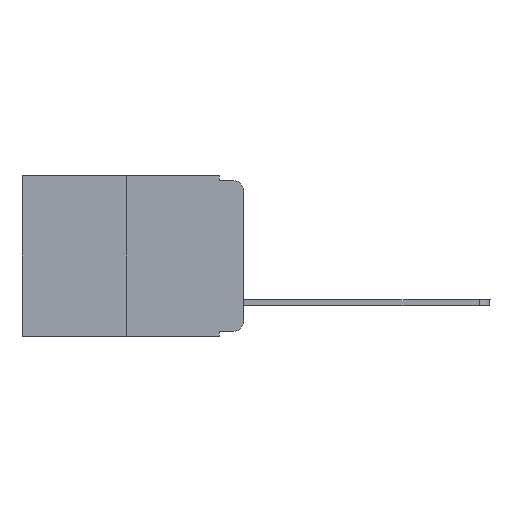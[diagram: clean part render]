
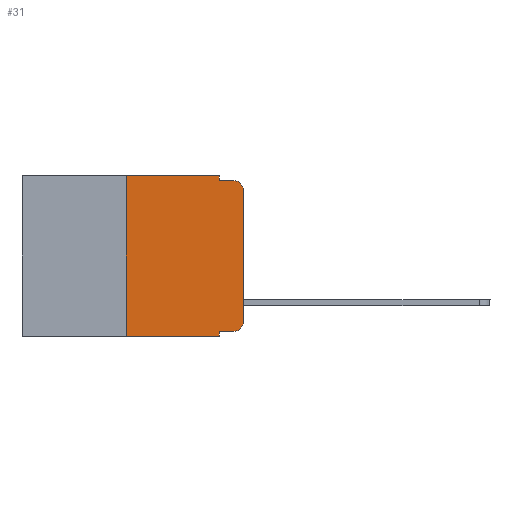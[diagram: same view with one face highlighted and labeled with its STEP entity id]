
A CAD part, left-side view. The second image highlights one B-rep face of the part: STEP entity #31.
In plain terms, the highlighted planar face has unit normal (-1, 0, 0).
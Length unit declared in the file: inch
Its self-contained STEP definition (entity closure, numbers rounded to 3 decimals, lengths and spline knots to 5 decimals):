
#31 = ADVANCED_FACE ( 'NONE', ( #7737 ), #12388, .F. ) ;
#582 = CARTESIAN_POINT ( 'NONE',  ( 0., 0.051, -0.333 ) ) ;
#737 = VECTOR ( 'NONE', #14492, 39.37008 ) ;
#1043 = AXIS2_PLACEMENT_3D ( 'NONE', #17936, #7606, #17555 ) ;
#1588 = VERTEX_POINT ( 'NONE', #3294 ) ;
#1659 = EDGE_CURVE ( 'NONE', #9934, #6963, #11977, .T. ) ;
#2437 = LINE ( 'NONE', #8331, #12179 ) ;
#2709 = VERTEX_POINT ( 'NONE', #6321 ) ;
#2889 = CARTESIAN_POINT ( 'NONE',  ( 0., 0.473, -0.343 ) ) ;
#2942 = EDGE_CURVE ( 'NONE', #1588, #2977, #2437, .T. ) ;
#2977 = VERTEX_POINT ( 'NONE', #8709 ) ;
#3294 = CARTESIAN_POINT ( 'NONE',  ( 0., 0.051, -0.01 ) ) ;
#3409 = EDGE_CURVE ( 'NONE', #14223, #2709, #3972, .T. ) ;
#3478 = CARTESIAN_POINT ( 'NONE',  ( 0., 0., -0.03 ) ) ;
#3717 = CARTESIAN_POINT ( 'NONE',  ( 0., 0.25, 0. ) ) ;
#3972 = LINE ( 'NONE', #8587, #737 ) ;
#4462 = VECTOR ( 'NONE', #11658, 39.37008 ) ;
#4590 = EDGE_LOOP ( 'NONE', ( #5591, #15551, #16948, #12544, #4795, #11921, #11874, #5206, #12717, #8616 ) ) ;
#4795 = ORIENTED_EDGE ( 'NONE', *, *, #3409, .F. ) ;
#4999 = VERTEX_POINT ( 'NONE', #13820 ) ;
#5048 = CARTESIAN_POINT ( 'NONE',  ( 0., 0.473, 0. ) ) ;
#5103 = AXIS2_PLACEMENT_3D ( 'NONE', #16320, #8453, #9553 ) ;
#5129 = VERTEX_POINT ( 'NONE', #3478 ) ;
#5206 = ORIENTED_EDGE ( 'NONE', *, *, #6275, .F. ) ;
#5591 = ORIENTED_EDGE ( 'NONE', *, *, #17825, .T. ) ;
#5823 = EDGE_CURVE ( 'NONE', #11253, #9641, #11933, .T. ) ;
#5833 = CARTESIAN_POINT ( 'NONE',  ( 0., 0.02, -0.333 ) ) ;
#5845 = LINE ( 'NONE', #10463, #8796 ) ;
#6021 = CIRCLE ( 'NONE', #5103, 0.02 ) ;
#6275 = EDGE_CURVE ( 'NONE', #11253, #6963, #5845, .T. ) ;
#6321 = CARTESIAN_POINT ( 'NONE',  ( 0., 0.051, 0. ) ) ;
#6918 = CIRCLE ( 'NONE', #1043, 0.02 ) ;
#6963 = VERTEX_POINT ( 'NONE', #8038 ) ;
#7606 = DIRECTION ( 'NONE',  ( -1., 0., 0. ) ) ;
#7737 = FACE_OUTER_BOUND ( 'NONE', #4590, .T. ) ;
#7942 = DIRECTION ( 'NONE',  ( 1., 0., 0. ) ) ;
#8038 = CARTESIAN_POINT ( 'NONE',  ( 0., 0.051, -0.343 ) ) ;
#8331 = CARTESIAN_POINT ( 'NONE',  ( 0., 0.051, -0.01 ) ) ;
#8453 = DIRECTION ( 'NONE',  ( -1., 0., 0. ) ) ;
#8587 = CARTESIAN_POINT ( 'NONE',  ( 0., 0.473, 0. ) ) ;
#8616 = ORIENTED_EDGE ( 'NONE', *, *, #17842, .T. ) ;
#8709 = CARTESIAN_POINT ( 'NONE',  ( 0., 0.02, -0.01 ) ) ;
#8710 = AXIS2_PLACEMENT_3D ( 'NONE', #5048, #7942, #13839 ) ;
#8762 = CARTESIAN_POINT ( 'NONE',  ( 0., 0., 0. ) ) ;
#8796 = VECTOR ( 'NONE', #10268, 39.37008 ) ;
#9553 = DIRECTION ( 'NONE',  ( 0., 0., -1. ) ) ;
#9641 = VERTEX_POINT ( 'NONE', #5833 ) ;
#9780 = LINE ( 'NONE', #11407, #12116 ) ;
#9934 = VERTEX_POINT ( 'NONE', #17192 ) ;
#10268 = DIRECTION ( 'NONE',  ( 0., 0., -1. ) ) ;
#10463 = CARTESIAN_POINT ( 'NONE',  ( 0., 0.051, 0. ) ) ;
#10466 = DIRECTION ( 'NONE',  ( 0., -1., 0. ) ) ;
#10836 = CARTESIAN_POINT ( 'NONE',  ( 0., 0.051, -0.333 ) ) ;
#11253 = VERTEX_POINT ( 'NONE', #582 ) ;
#11407 = CARTESIAN_POINT ( 'NONE',  ( 0., 0.051, 0. ) ) ;
#11658 = DIRECTION ( 'NONE',  ( 0., 0., 1. ) ) ;
#11874 = ORIENTED_EDGE ( 'NONE', *, *, #1659, .T. ) ;
#11880 = CARTESIAN_POINT ( 'NONE',  ( 0., 0.25, 0. ) ) ;
#11921 = ORIENTED_EDGE ( 'NONE', *, *, #17432, .F. ) ;
#11933 = LINE ( 'NONE', #10836, #13160 ) ;
#11960 = LINE ( 'NONE', #8762, #4462 ) ;
#11977 = LINE ( 'NONE', #2889, #13785 ) ;
#12116 = VECTOR ( 'NONE', #14318, 39.37008 ) ;
#12179 = VECTOR ( 'NONE', #14235, 39.37008 ) ;
#12388 = PLANE ( 'NONE',  #8710 ) ;
#12544 = ORIENTED_EDGE ( 'NONE', *, *, #13841, .F. ) ;
#12717 = ORIENTED_EDGE ( 'NONE', *, *, #5823, .T. ) ;
#13160 = VECTOR ( 'NONE', #10466, 39.37008 ) ;
#13785 = VECTOR ( 'NONE', #14786, 39.37008 ) ;
#13820 = CARTESIAN_POINT ( 'NONE',  ( 0., 0., -0.313 ) ) ;
#13839 = DIRECTION ( 'NONE',  ( 0., 0., -1. ) ) ;
#13841 = EDGE_CURVE ( 'NONE', #2709, #1588, #9780, .T. ) ;
#14223 = VERTEX_POINT ( 'NONE', #3717 ) ;
#14235 = DIRECTION ( 'NONE',  ( 0., -1., 0. ) ) ;
#14318 = DIRECTION ( 'NONE',  ( 0., 0., -1. ) ) ;
#14492 = DIRECTION ( 'NONE',  ( 0., -1., 0. ) ) ;
#14786 = DIRECTION ( 'NONE',  ( 0., -1., 0. ) ) ;
#15551 = ORIENTED_EDGE ( 'NONE', *, *, #18318, .T. ) ;
#16320 = CARTESIAN_POINT ( 'NONE',  ( 0., 0.02, -0.03 ) ) ;
#16412 = DIRECTION ( 'NONE',  ( 0., 0., 1. ) ) ;
#16948 = ORIENTED_EDGE ( 'NONE', *, *, #2942, .F. ) ;
#17192 = CARTESIAN_POINT ( 'NONE',  ( 0., 0.25, -0.343 ) ) ;
#17432 = EDGE_CURVE ( 'NONE', #9934, #14223, #17963, .T. ) ;
#17555 = DIRECTION ( 'NONE',  ( 0., 0., -1. ) ) ;
#17825 = EDGE_CURVE ( 'NONE', #4999, #5129, #11960, .T. ) ;
#17842 = EDGE_CURVE ( 'NONE', #9641, #4999, #6918, .T. ) ;
#17936 = CARTESIAN_POINT ( 'NONE',  ( 0., 0.02, -0.313 ) ) ;
#17963 = LINE ( 'NONE', #11880, #18684 ) ;
#18318 = EDGE_CURVE ( 'NONE', #5129, #2977, #6021, .T. ) ;
#18684 = VECTOR ( 'NONE', #16412, 39.37008 ) ;
